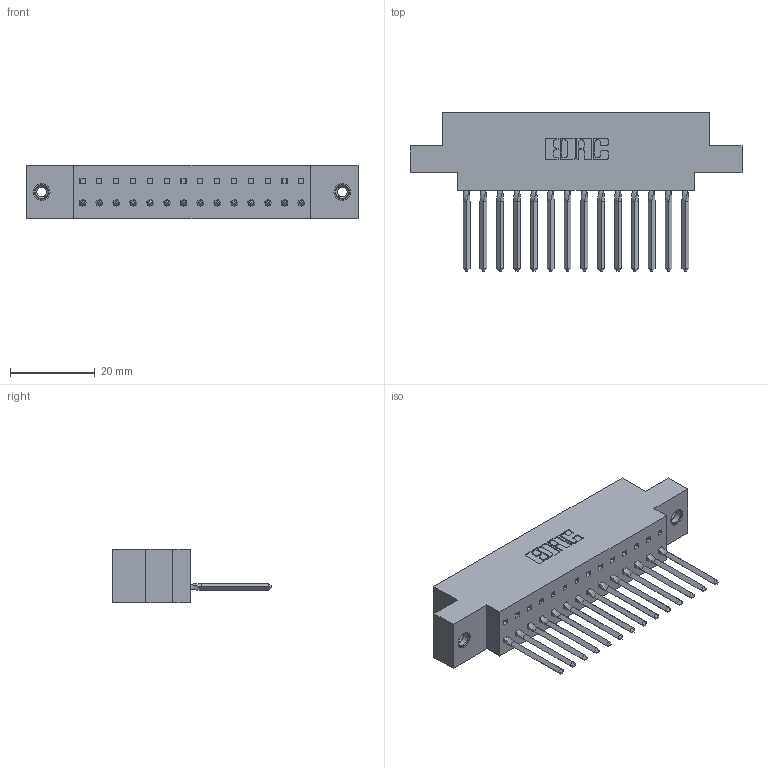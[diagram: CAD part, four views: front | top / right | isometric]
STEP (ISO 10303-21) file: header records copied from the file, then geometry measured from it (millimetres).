
FILE_DESCRIPTION (( 'STEP AP203' ), '1' );
FILE_NAME ('317-014-541-678.STEP', '2020-02-27T14:39:40', ( '' ), ( '' ), 'SwSTEP 2.0', 'SolidWorks 2016', '' );
FILE_SCHEMA (( 'CONFIG_CONTROL_DESIGN' ));
Length unit declared in the file: inch
Products named in the file (4): 345-250-001_345-250-003-102; 317-014-541-678; 317-290-002_541; 317 Part_.156 Dia - TI
Assembly tree (17 placements, depth 2):
  317-014-541-678
    317 Part_.156 Dia - TI
    317-290-002_541  x14
    345-250-001_345-250-003-102  x2
Bounding box: 78.18 x 37.34 x 12.7 mm (x, y, z)
Volume: 11810.9 mm3; surface area: 15777.6 mm2
Topology: 17 solids, 17 shells, 2290 faces, 6487 edges, 4214 vertices
Faces by surface type: plane 1826, cylinder 392, bspline 56, cone 12, torus 4
Entity records: 26429 total; most frequent: CARTESIAN_POINT 5294, ORIENTED_EDGE 4554, DIRECTION 3763, EDGE_CURVE 2277, LINE 1893, VECTOR 1893, VERTEX_POINT 1506, AXIS2_PLACEMENT_3D 935
